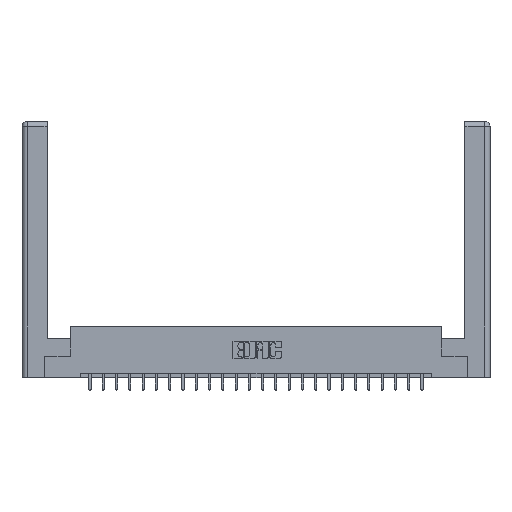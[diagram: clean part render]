
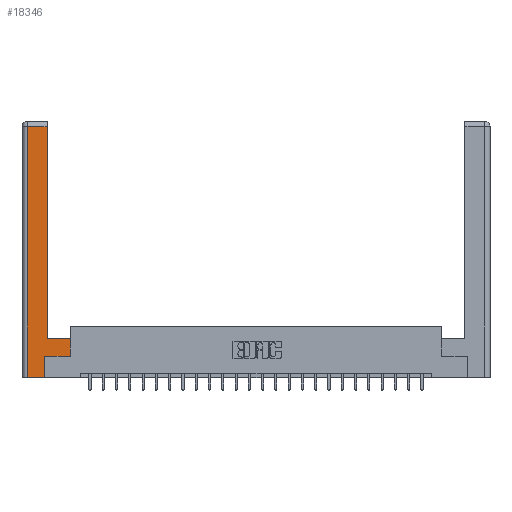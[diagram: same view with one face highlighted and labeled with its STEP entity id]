
A CAD part, top view. The second image highlights one B-rep face of the part: STEP entity #18346.
In plain terms, the highlighted planar face has unit normal (0, 0, 1).
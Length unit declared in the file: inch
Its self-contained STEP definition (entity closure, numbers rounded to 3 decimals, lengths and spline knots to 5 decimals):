
#901 = DIRECTION ( 'NONE',  ( 1., 0., 0. ) ) ;
#1841 = DIRECTION ( 'NONE',  ( -1., 0., 0. ) ) ;
#2719 = VECTOR ( 'NONE', #14217, 39.37008 ) ;
#3846 = PLANE ( 'NONE',  #15000 ) ;
#4009 = DIRECTION ( 'NONE',  ( 0., 1., 0. ) ) ;
#4917 = ORIENTED_EDGE ( 'NONE', *, *, #16651, .T. ) ;
#5266 = CARTESIAN_POINT ( 'NONE',  ( 0.265, 0.245, 0. ) ) ;
#5536 = DIRECTION ( 'NONE',  ( 0., 0., -1. ) ) ;
#5866 = CARTESIAN_POINT ( 'NONE',  ( 0.565, 0.245, 0. ) ) ;
#5923 = CARTESIAN_POINT ( 'NONE',  ( 0.0615, 2.94, 0. ) ) ;
#6325 = CARTESIAN_POINT ( 'NONE',  ( 0.0615, 0., 0. ) ) ;
#6441 = CARTESIAN_POINT ( 'NONE',  ( 0.565, 0.45, 0. ) ) ;
#6619 = ORIENTED_EDGE ( 'NONE', *, *, #23726, .T. ) ;
#6865 = EDGE_CURVE ( 'NONE', #21975, #8746, #23216, .T. ) ;
#6892 = CARTESIAN_POINT ( 'NONE',  ( 0.0615, 0., 0. ) ) ;
#7193 = ORIENTED_EDGE ( 'NONE', *, *, #7649, .T. ) ;
#7649 = EDGE_CURVE ( 'NONE', #20695, #24229, #8704, .T. ) ;
#7820 = VECTOR ( 'NONE', #4009, 39.37008 ) ;
#8704 = LINE ( 'NONE', #6892, #16266 ) ;
#8746 = VERTEX_POINT ( 'NONE', #6441 ) ;
#9670 = EDGE_CURVE ( 'NONE', #20052, #12129, #17124, .T. ) ;
#10076 = VECTOR ( 'NONE', #22412, 39.37008 ) ;
#10485 = CARTESIAN_POINT ( 'NONE',  ( 0.295, 2.94, 0. ) ) ;
#11080 = ORIENTED_EDGE ( 'NONE', *, *, #14581, .T. ) ;
#11308 = CARTESIAN_POINT ( 'NONE',  ( 0.295, 3., 0. ) ) ;
#11493 = VECTOR ( 'NONE', #12909, 39.37008 ) ;
#12129 = VERTEX_POINT ( 'NONE', #10485 ) ;
#12225 = CARTESIAN_POINT ( 'NONE',  ( 0.0615, 2.94, 0. ) ) ;
#12340 = DIRECTION ( 'NONE',  ( 0., 1., 0. ) ) ;
#12375 = VECTOR ( 'NONE', #901, 39.37008 ) ;
#12817 = CARTESIAN_POINT ( 'NONE',  ( 0.295, 0.45, 0. ) ) ;
#12909 = DIRECTION ( 'NONE',  ( 0., 1., 0. ) ) ;
#13691 = CARTESIAN_POINT ( 'NONE',  ( 0.565, 0.45, 0. ) ) ;
#14217 = DIRECTION ( 'NONE',  ( 1., 0., 0. ) ) ;
#14501 = DIRECTION ( 'NONE',  ( 0., -1., 0. ) ) ;
#14547 = VERTEX_POINT ( 'NONE', #21988 ) ;
#14581 = EDGE_CURVE ( 'NONE', #8746, #20052, #18205, .T. ) ;
#14973 = FACE_OUTER_BOUND ( 'NONE', #15781, .T. ) ;
#15000 = AXIS2_PLACEMENT_3D ( 'NONE', #19175, #5536, #1841 ) ;
#15298 = ORIENTED_EDGE ( 'NONE', *, *, #6865, .T. ) ;
#15467 = VERTEX_POINT ( 'NONE', #21370 ) ;
#15781 = EDGE_LOOP ( 'NONE', ( #19829, #6619, #7193, #4917, #22444, #20917, #15298, #11080 ) ) ;
#15979 = LINE ( 'NONE', #17766, #2719 ) ;
#16121 = CARTESIAN_POINT ( 'NONE',  ( 0.565, 0.245, 0. ) ) ;
#16195 = EDGE_CURVE ( 'NONE', #15467, #21975, #19929, .T. ) ;
#16266 = VECTOR ( 'NONE', #14501, 39.37008 ) ;
#16454 = EDGE_CURVE ( 'NONE', #14547, #15467, #22615, .T. ) ;
#16651 = EDGE_CURVE ( 'NONE', #24229, #14547, #15979, .T. ) ;
#17124 = LINE ( 'NONE', #11308, #20135 ) ;
#17766 = CARTESIAN_POINT ( 'NONE',  ( 0.265, 0., 0. ) ) ;
#18042 = DIRECTION ( 'NONE',  ( -1., 0., 0. ) ) ;
#18205 = LINE ( 'NONE', #20474, #10076 ) ;
#18346 = ADVANCED_FACE ( 'NONE', ( #14973 ), #3846, .F. ) ;
#19175 = CARTESIAN_POINT ( 'NONE',  ( 0., 0., 0. ) ) ;
#19829 = ORIENTED_EDGE ( 'NONE', *, *, #9670, .T. ) ;
#19929 = LINE ( 'NONE', #16121, #12375 ) ;
#20052 = VERTEX_POINT ( 'NONE', #12817 ) ;
#20135 = VECTOR ( 'NONE', #12340, 39.37008 ) ;
#20474 = CARTESIAN_POINT ( 'NONE',  ( 0.295, 0.45, 0. ) ) ;
#20695 = VERTEX_POINT ( 'NONE', #12225 ) ;
#20917 = ORIENTED_EDGE ( 'NONE', *, *, #16195, .T. ) ;
#21370 = CARTESIAN_POINT ( 'NONE',  ( 0.265, 0.245, 0. ) ) ;
#21975 = VERTEX_POINT ( 'NONE', #5866 ) ;
#21988 = CARTESIAN_POINT ( 'NONE',  ( 0.265, 0., 0. ) ) ;
#22412 = DIRECTION ( 'NONE',  ( -1., 0., 0. ) ) ;
#22444 = ORIENTED_EDGE ( 'NONE', *, *, #16454, .T. ) ;
#22615 = LINE ( 'NONE', #5266, #11493 ) ;
#23216 = LINE ( 'NONE', #13691, #7820 ) ;
#23726 = EDGE_CURVE ( 'NONE', #12129, #20695, #24611, .T. ) ;
#23997 = VECTOR ( 'NONE', #18042, 39.37008 ) ;
#24229 = VERTEX_POINT ( 'NONE', #6325 ) ;
#24611 = LINE ( 'NONE', #5923, #23997 ) ;
